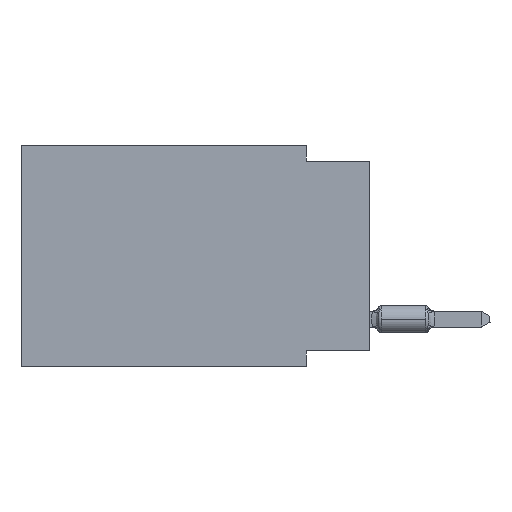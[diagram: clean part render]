
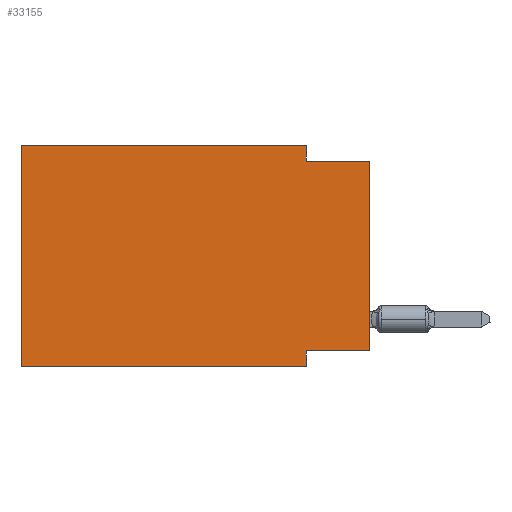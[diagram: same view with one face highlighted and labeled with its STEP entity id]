
A CAD part, left-side view. The second image highlights one B-rep face of the part: STEP entity #33155.
In plain terms, the highlighted planar face has unit normal (-1, 0, 0).
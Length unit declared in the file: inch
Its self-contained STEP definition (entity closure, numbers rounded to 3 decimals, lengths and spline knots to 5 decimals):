
#276 = ORIENTED_EDGE ( 'NONE', *, *, #5378, .F. ) ;
#1647 = ORIENTED_EDGE ( 'NONE', *, *, #10291, .F. ) ;
#2369 = CARTESIAN_POINT ( 'NONE',  ( 0., 0.1, 0. ) ) ;
#2895 = AXIS2_PLACEMENT_3D ( 'NONE', #19086, #53409, #14859 ) ;
#3221 = DIRECTION ( 'NONE',  ( 0., -1., 0. ) ) ;
#3297 = VERTEX_POINT ( 'NONE', #28308 ) ;
#4141 = VECTOR ( 'NONE', #49421, 39.37008 ) ;
#5378 = EDGE_CURVE ( 'NONE', #42634, #14489, #43096, .T. ) ;
#5393 = CARTESIAN_POINT ( 'NONE',  ( 0., 0.55, 0. ) ) ;
#6434 = EDGE_CURVE ( 'NONE', #48168, #14489, #33550, .T. ) ;
#8436 = CARTESIAN_POINT ( 'NONE',  ( 0., 0.1, -0.35 ) ) ;
#9114 = CARTESIAN_POINT ( 'NONE',  ( 0., 0.55, 0. ) ) ;
#9887 = EDGE_CURVE ( 'NONE', #3297, #43755, #16270, .T. ) ;
#10291 = EDGE_CURVE ( 'NONE', #49482, #43755, #24398, .T. ) ;
#10644 = LINE ( 'NONE', #23896, #27760 ) ;
#10843 = CARTESIAN_POINT ( 'NONE',  ( 0., 0., -0.025 ) ) ;
#12379 = DIRECTION ( 'NONE',  ( 0., 0., -1. ) ) ;
#13624 = DIRECTION ( 'NONE',  ( 0., 0., -1. ) ) ;
#14068 = DIRECTION ( 'NONE',  ( 0., 1., 0. ) ) ;
#14401 = CARTESIAN_POINT ( 'NONE',  ( 0., 0.1, -0.325 ) ) ;
#14489 = VERTEX_POINT ( 'NONE', #34160 ) ;
#14580 = PLANE ( 'NONE',  #2895 ) ;
#14859 = DIRECTION ( 'NONE',  ( 0., 0., -1. ) ) ;
#15998 = CARTESIAN_POINT ( 'NONE',  ( 0., 0., 0. ) ) ;
#16209 = CARTESIAN_POINT ( 'NONE',  ( 0., 0., -0.025 ) ) ;
#16270 = LINE ( 'NONE', #15998, #41551 ) ;
#16370 = VECTOR ( 'NONE', #3221, 39.37008 ) ;
#17685 = VERTEX_POINT ( 'NONE', #2369 ) ;
#17797 = VECTOR ( 'NONE', #13624, 39.37008 ) ;
#17821 = ORIENTED_EDGE ( 'NONE', *, *, #9887, .T. ) ;
#19086 = CARTESIAN_POINT ( 'NONE',  ( 0., 0.55, 0. ) ) ;
#22425 = ORIENTED_EDGE ( 'NONE', *, *, #39388, .F. ) ;
#23429 = ORIENTED_EDGE ( 'NONE', *, *, #54098, .F. ) ;
#23582 = FACE_OUTER_BOUND ( 'NONE', #48580, .T. ) ;
#23896 = CARTESIAN_POINT ( 'NONE',  ( 0., 0., -0.325 ) ) ;
#24085 = CARTESIAN_POINT ( 'NONE',  ( 0., 0.55, 0. ) ) ;
#24398 = LINE ( 'NONE', #16209, #16370 ) ;
#27760 = VECTOR ( 'NONE', #14068, 39.37008 ) ;
#27894 = ORIENTED_EDGE ( 'NONE', *, *, #40745, .F. ) ;
#28308 = CARTESIAN_POINT ( 'NONE',  ( 0., 0., -0.325 ) ) ;
#28977 = ORIENTED_EDGE ( 'NONE', *, *, #48332, .F. ) ;
#29124 = ORIENTED_EDGE ( 'NONE', *, *, #6434, .T. ) ;
#31602 = DIRECTION ( 'NONE',  ( 0., -1., 0. ) ) ;
#31649 = LINE ( 'NONE', #48265, #17797 ) ;
#32356 = DIRECTION ( 'NONE',  ( 0., 0., 1. ) ) ;
#32995 = DIRECTION ( 'NONE',  ( 0., -1., 0. ) ) ;
#33155 = ADVANCED_FACE ( 'NONE', ( #23582 ), #14580, .F. ) ;
#33550 = LINE ( 'NONE', #49596, #40354 ) ;
#34160 = CARTESIAN_POINT ( 'NONE',  ( 0., 0.1, -0.35 ) ) ;
#34730 = LINE ( 'NONE', #5393, #47901 ) ;
#34924 = CARTESIAN_POINT ( 'NONE',  ( 0., 0.55, -0.35 ) ) ;
#36700 = VECTOR ( 'NONE', #12379, 39.37008 ) ;
#39388 = EDGE_CURVE ( 'NONE', #48168, #40699, #40725, .T. ) ;
#40354 = VECTOR ( 'NONE', #32995, 39.37008 ) ;
#40699 = VERTEX_POINT ( 'NONE', #9114 ) ;
#40725 = LINE ( 'NONE', #24085, #4141 ) ;
#40745 = EDGE_CURVE ( 'NONE', #17685, #49482, #31649, .T. ) ;
#41551 = VECTOR ( 'NONE', #32356, 39.37008 ) ;
#42634 = VERTEX_POINT ( 'NONE', #14401 ) ;
#43096 = LINE ( 'NONE', #8436, #36700 ) ;
#43755 = VERTEX_POINT ( 'NONE', #10843 ) ;
#47590 = CARTESIAN_POINT ( 'NONE',  ( 0., 0.1, -0.025 ) ) ;
#47901 = VECTOR ( 'NONE', #31602, 39.37008 ) ;
#48168 = VERTEX_POINT ( 'NONE', #34924 ) ;
#48265 = CARTESIAN_POINT ( 'NONE',  ( 0., 0.1, 0. ) ) ;
#48332 = EDGE_CURVE ( 'NONE', #3297, #42634, #10644, .T. ) ;
#48580 = EDGE_LOOP ( 'NONE', ( #17821, #1647, #27894, #23429, #22425, #29124, #276, #28977 ) ) ;
#49421 = DIRECTION ( 'NONE',  ( 0., 0., 1. ) ) ;
#49482 = VERTEX_POINT ( 'NONE', #47590 ) ;
#49596 = CARTESIAN_POINT ( 'NONE',  ( 0., 0.55, -0.35 ) ) ;
#53409 = DIRECTION ( 'NONE',  ( 1., 0., 0. ) ) ;
#54098 = EDGE_CURVE ( 'NONE', #40699, #17685, #34730, .T. ) ;
